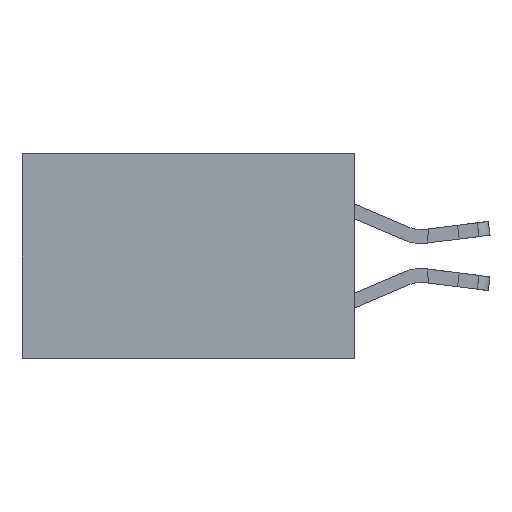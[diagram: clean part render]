
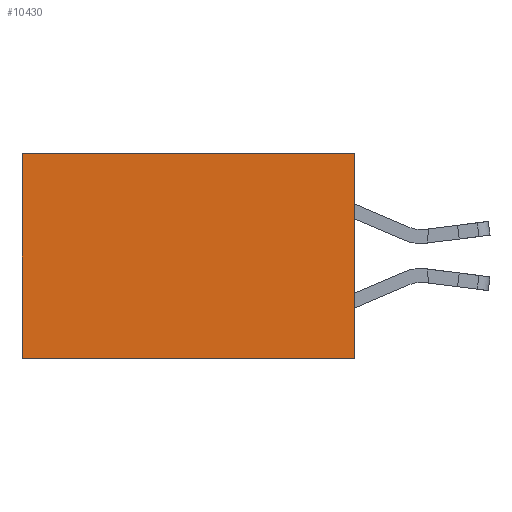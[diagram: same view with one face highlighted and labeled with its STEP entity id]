
A CAD part, left-side view. The second image highlights one B-rep face of the part: STEP entity #10430.
In plain terms, the highlighted planar face has unit normal (-1, 0, 0).
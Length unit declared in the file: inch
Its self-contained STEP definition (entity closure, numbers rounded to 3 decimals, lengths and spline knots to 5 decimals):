
#5 = EDGE_CURVE ( 'NONE', #3682, #21816, #5117, .T. ) ;
#851 = CARTESIAN_POINT ( 'NONE',  ( 0.2615, 0., -0.37 ) ) ;
#1859 = VECTOR ( 'NONE', #10107, 39.37008 ) ;
#2158 = EDGE_CURVE ( 'NONE', #17758, #21816, #11697, .T. ) ;
#2428 = VECTOR ( 'NONE', #10116, 39.37008 ) ;
#2681 = CARTESIAN_POINT ( 'NONE',  ( 0.2615, 0., -0.37 ) ) ;
#2919 = CARTESIAN_POINT ( 'NONE',  ( 0.2615, 0.6, -0.37 ) ) ;
#3192 = PLANE ( 'NONE',  #3629 ) ;
#3360 = VERTEX_POINT ( 'NONE', #14288 ) ;
#3484 = ORIENTED_EDGE ( 'NONE', *, *, #5, .T. ) ;
#3629 = AXIS2_PLACEMENT_3D ( 'NONE', #851, #13328, #8079 ) ;
#3682 = VERTEX_POINT ( 'NONE', #11704 ) ;
#4544 = CARTESIAN_POINT ( 'NONE',  ( 0.2615, 0., 0. ) ) ;
#5117 = LINE ( 'NONE', #6611, #1859 ) ;
#6611 = CARTESIAN_POINT ( 'NONE',  ( 0.2615, 0.6, -0.37 ) ) ;
#8076 = EDGE_CURVE ( 'NONE', #3360, #3682, #15239, .T. ) ;
#8079 = DIRECTION ( 'NONE',  ( 0., 0., -1. ) ) ;
#8250 = ORIENTED_EDGE ( 'NONE', *, *, #19048, .F. ) ;
#10107 = DIRECTION ( 'NONE',  ( 0., 0., -1. ) ) ;
#10116 = DIRECTION ( 'NONE',  ( 0., 1., 0. ) ) ;
#10303 = ORIENTED_EDGE ( 'NONE', *, *, #8076, .T. ) ;
#10430 = ADVANCED_FACE ( 'NONE', ( #16920 ), #3192, .F. ) ;
#10523 = EDGE_LOOP ( 'NONE', ( #3484, #17526, #8250, #10303 ) ) ;
#11652 = CARTESIAN_POINT ( 'NONE',  ( 0.2615, 0., -0.37 ) ) ;
#11697 = LINE ( 'NONE', #15175, #12476 ) ;
#11704 = CARTESIAN_POINT ( 'NONE',  ( 0.2615, 0.6, 0. ) ) ;
#12476 = VECTOR ( 'NONE', #22049, 39.37008 ) ;
#13328 = DIRECTION ( 'NONE',  ( 1., 0., 0. ) ) ;
#14288 = CARTESIAN_POINT ( 'NONE',  ( 0.2615, 0., 0. ) ) ;
#14468 = VECTOR ( 'NONE', #17230, 39.37008 ) ;
#15037 = LINE ( 'NONE', #11652, #14468 ) ;
#15175 = CARTESIAN_POINT ( 'NONE',  ( 0.2615, 0., -0.37 ) ) ;
#15239 = LINE ( 'NONE', #4544, #2428 ) ;
#16920 = FACE_OUTER_BOUND ( 'NONE', #10523, .T. ) ;
#17230 = DIRECTION ( 'NONE',  ( 0., 0., -1. ) ) ;
#17526 = ORIENTED_EDGE ( 'NONE', *, *, #2158, .F. ) ;
#17758 = VERTEX_POINT ( 'NONE', #2681 ) ;
#19048 = EDGE_CURVE ( 'NONE', #3360, #17758, #15037, .T. ) ;
#21816 = VERTEX_POINT ( 'NONE', #2919 ) ;
#22049 = DIRECTION ( 'NONE',  ( 0., 1., 0. ) ) ;
